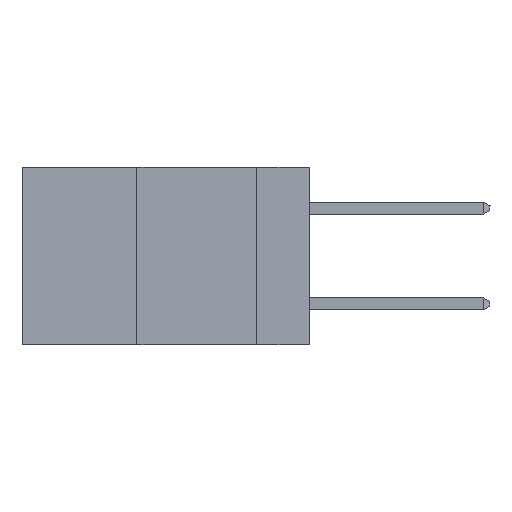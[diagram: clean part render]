
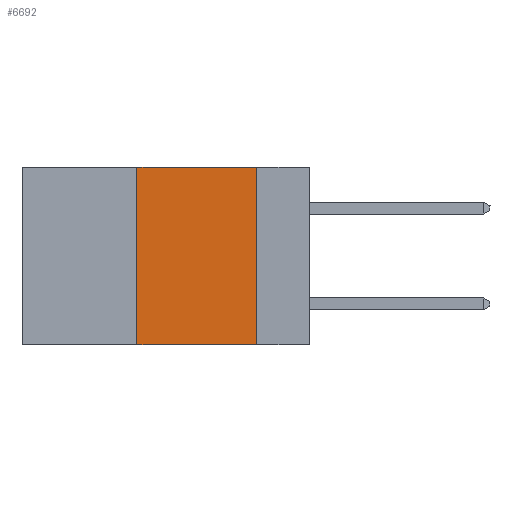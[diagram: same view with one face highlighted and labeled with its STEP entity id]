
A CAD part, left-side view. The second image highlights one B-rep face of the part: STEP entity #6692.
In plain terms, the highlighted planar face has unit normal (-1, 0, 0).
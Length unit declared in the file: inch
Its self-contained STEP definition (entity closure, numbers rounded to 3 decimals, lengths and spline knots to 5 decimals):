
#1557 = AXIS2_PLACEMENT_3D ( 'NONE', #8762, #5522, #7168 ) ;
#2781 = VECTOR ( 'NONE', #20237, 39.37008 ) ;
#3155 = VERTEX_POINT ( 'NONE', #19841 ) ;
#3499 = VECTOR ( 'NONE', #6498, 39.37008 ) ;
#3591 = VERTEX_POINT ( 'NONE', #12774 ) ;
#4310 = VECTOR ( 'NONE', #5867, 39.37008 ) ;
#4592 = PLANE ( 'NONE',  #1557 ) ;
#4815 = LINE ( 'NONE', #4840, #3499 ) ;
#4840 = CARTESIAN_POINT ( 'NONE',  ( 0., 0.11, 0. ) ) ;
#4958 = EDGE_CURVE ( 'NONE', #3155, #14461, #6649, .T. ) ;
#5522 = DIRECTION ( 'NONE',  ( 1., 0., 0. ) ) ;
#5867 = DIRECTION ( 'NONE',  ( 0., -1., 0. ) ) ;
#6006 = ORIENTED_EDGE ( 'NONE', *, *, #9804, .F. ) ;
#6130 = CARTESIAN_POINT ( 'NONE',  ( 0., 0.6, 0. ) ) ;
#6197 = DIRECTION ( 'NONE',  ( 0., -1., 0. ) ) ;
#6498 = DIRECTION ( 'NONE',  ( 0., 0., -1. ) ) ;
#6649 = LINE ( 'NONE', #16904, #2781 ) ;
#6692 = ADVANCED_FACE ( 'NONE', ( #10151 ), #4592, .F. ) ;
#7168 = DIRECTION ( 'NONE',  ( 0., 0., -1. ) ) ;
#8762 = CARTESIAN_POINT ( 'NONE',  ( 0., 0.6, 0. ) ) ;
#9804 = EDGE_CURVE ( 'NONE', #14461, #3591, #19626, .T. ) ;
#10151 = FACE_OUTER_BOUND ( 'NONE', #17133, .T. ) ;
#11437 = EDGE_CURVE ( 'NONE', #3155, #16797, #20049, .T. ) ;
#12141 = CARTESIAN_POINT ( 'NONE',  ( 0., 0.36, 0. ) ) ;
#12336 = CARTESIAN_POINT ( 'NONE',  ( 0., 0.11, -0.37 ) ) ;
#12774 = CARTESIAN_POINT ( 'NONE',  ( 0., 0.11, 0. ) ) ;
#13193 = ORIENTED_EDGE ( 'NONE', *, *, #11437, .T. ) ;
#14461 = VERTEX_POINT ( 'NONE', #12141 ) ;
#15188 = VECTOR ( 'NONE', #6197, 39.37008 ) ;
#15670 = ORIENTED_EDGE ( 'NONE', *, *, #4958, .F. ) ;
#16797 = VERTEX_POINT ( 'NONE', #12336 ) ;
#16904 = CARTESIAN_POINT ( 'NONE',  ( 0., 0.36, 0. ) ) ;
#17133 = EDGE_LOOP ( 'NONE', ( #20846, #6006, #15670, #13193 ) ) ;
#18951 = CARTESIAN_POINT ( 'NONE',  ( 0., 0.6, -0.37 ) ) ;
#19216 = EDGE_CURVE ( 'NONE', #3591, #16797, #4815, .T. ) ;
#19626 = LINE ( 'NONE', #6130, #15188 ) ;
#19841 = CARTESIAN_POINT ( 'NONE',  ( 0., 0.36, -0.37 ) ) ;
#20049 = LINE ( 'NONE', #18951, #4310 ) ;
#20237 = DIRECTION ( 'NONE',  ( 0., 0., 1. ) ) ;
#20846 = ORIENTED_EDGE ( 'NONE', *, *, #19216, .F. ) ;
